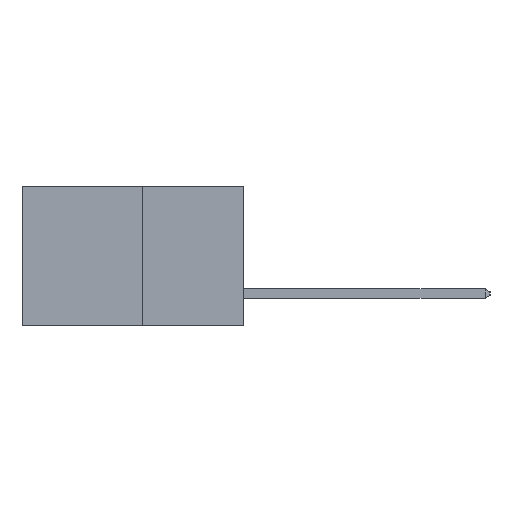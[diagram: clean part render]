
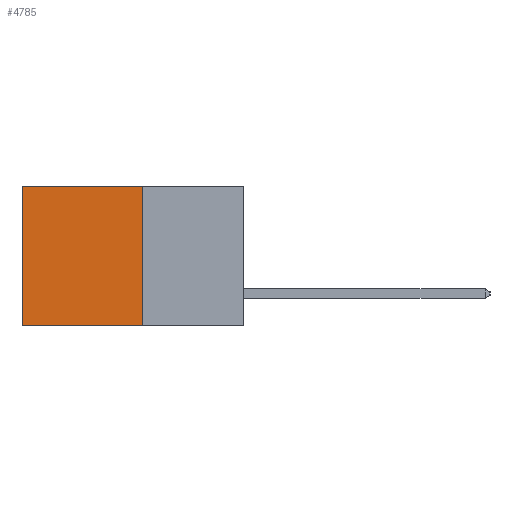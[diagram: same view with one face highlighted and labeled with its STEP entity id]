
A CAD part, left-side view. The second image highlights one B-rep face of the part: STEP entity #4785.
In plain terms, the highlighted planar face has unit normal (-1, 0, 0).
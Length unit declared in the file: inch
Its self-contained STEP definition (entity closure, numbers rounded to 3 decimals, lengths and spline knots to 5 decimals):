
#195 = CARTESIAN_POINT ( 'NONE',  ( 0.277, 0.27, -0.37 ) ) ;
#344 = CARTESIAN_POINT ( 'NONE',  ( 0.277, 0.27, -0.37 ) ) ;
#471 = VECTOR ( 'NONE', #12526, 39.37008 ) ;
#570 = CARTESIAN_POINT ( 'NONE',  ( 0.277, 0.27, -0.37 ) ) ;
#631 = DIRECTION ( 'NONE',  ( 0., 0., -1. ) ) ;
#1933 = VECTOR ( 'NONE', #4385, 39.37008 ) ;
#2387 = VERTEX_POINT ( 'NONE', #4511 ) ;
#2452 = EDGE_CURVE ( 'NONE', #9728, #2387, #16738, .T. ) ;
#2623 = CARTESIAN_POINT ( 'NONE',  ( 0.277, 0.27, 0. ) ) ;
#2943 = ORIENTED_EDGE ( 'NONE', *, *, #13602, .F. ) ;
#4385 = DIRECTION ( 'NONE',  ( 0., 0., -1. ) ) ;
#4511 = CARTESIAN_POINT ( 'NONE',  ( 0.277, 0.59, -0.37 ) ) ;
#4785 = ADVANCED_FACE ( 'NONE', ( #12011 ), #4787, .F. ) ;
#4787 = PLANE ( 'NONE',  #12995 ) ;
#5693 = CARTESIAN_POINT ( 'NONE',  ( 0.277, 0.59, 0. ) ) ;
#5812 = DIRECTION ( 'NONE',  ( 0., 1., 0. ) ) ;
#5904 = DIRECTION ( 'NONE',  ( 0., 1., 0. ) ) ;
#6356 = VECTOR ( 'NONE', #5812, 39.37008 ) ;
#7551 = ORIENTED_EDGE ( 'NONE', *, *, #17455, .F. ) ;
#8838 = VERTEX_POINT ( 'NONE', #2623 ) ;
#8875 = DIRECTION ( 'NONE',  ( 1., 0., 0. ) ) ;
#9028 = CARTESIAN_POINT ( 'NONE',  ( 0.277, 0.59, -0.37 ) ) ;
#9728 = VERTEX_POINT ( 'NONE', #5693 ) ;
#11382 = LINE ( 'NONE', #195, #471 ) ;
#11430 = ORIENTED_EDGE ( 'NONE', *, *, #17508, .T. ) ;
#11593 = VERTEX_POINT ( 'NONE', #344 ) ;
#12011 = FACE_OUTER_BOUND ( 'NONE', #15997, .T. ) ;
#12526 = DIRECTION ( 'NONE',  ( 0., 0., -1. ) ) ;
#12653 = CARTESIAN_POINT ( 'NONE',  ( 0.277, 0.27, 0. ) ) ;
#12907 = ORIENTED_EDGE ( 'NONE', *, *, #2452, .T. ) ;
#12995 = AXIS2_PLACEMENT_3D ( 'NONE', #570, #8875, #631 ) ;
#13602 = EDGE_CURVE ( 'NONE', #11593, #2387, #17070, .T. ) ;
#13719 = VECTOR ( 'NONE', #5904, 39.37008 ) ;
#14133 = LINE ( 'NONE', #12653, #13719 ) ;
#15223 = CARTESIAN_POINT ( 'NONE',  ( 0.277, 0.27, -0.37 ) ) ;
#15997 = EDGE_LOOP ( 'NONE', ( #12907, #2943, #7551, #11430 ) ) ;
#16738 = LINE ( 'NONE', #9028, #1933 ) ;
#17070 = LINE ( 'NONE', #15223, #6356 ) ;
#17455 = EDGE_CURVE ( 'NONE', #8838, #11593, #11382, .T. ) ;
#17508 = EDGE_CURVE ( 'NONE', #8838, #9728, #14133, .T. ) ;
